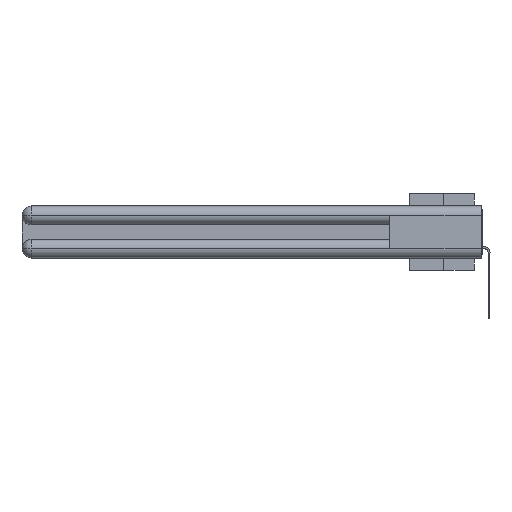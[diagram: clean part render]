
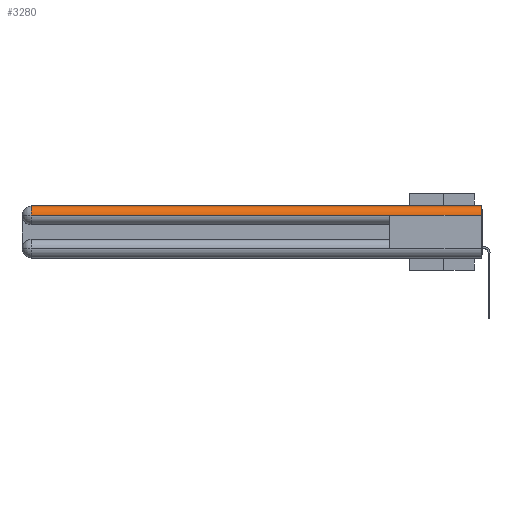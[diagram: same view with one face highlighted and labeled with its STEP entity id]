
A CAD part, left-side view. The second image highlights one B-rep face of the part: STEP entity #3280.
In plain terms, the highlighted cylindrical face has radius 1.562 mm (diameter 3.124 mm), a partial arc.
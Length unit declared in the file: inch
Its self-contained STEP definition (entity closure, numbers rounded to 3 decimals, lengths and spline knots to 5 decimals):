
#3280 = ADVANCED_FACE ( 'NONE', ( #16527 ), #18516, .T. ) ;
#3912 = ORIENTED_EDGE ( 'NONE', *, *, #4350, .F. ) ;
#4350 = EDGE_CURVE ( 'NONE', #36509, #22340, #38670, .T. ) ;
#5011 = DIRECTION ( 'NONE',  ( 0., -1., 0. ) ) ;
#5076 = VERTEX_POINT ( 'NONE', #14578 ) ;
#5189 = CARTESIAN_POINT ( 'NONE',  ( 0.0615, 2.94, 0. ) ) ;
#5241 = EDGE_CURVE ( 'NONE', #19698, #28461, #25313, .T. ) ;
#12131 = ORIENTED_EDGE ( 'NONE', *, *, #29637, .T. ) ;
#14134 = AXIS2_PLACEMENT_3D ( 'NONE', #31324, #15736, #18638 ) ;
#14578 = CARTESIAN_POINT ( 'NONE',  ( 0., 2.94, -0.0615 ) ) ;
#14628 = DIRECTION ( 'NONE',  ( 0., 1., 0. ) ) ;
#15383 = DIRECTION ( 'NONE',  ( 0., -1., 0. ) ) ;
#15409 = CIRCLE ( 'NONE', #25533, 0.0615 ) ;
#15736 = DIRECTION ( 'NONE',  ( 0., 1., 0. ) ) ;
#16182 = ORIENTED_EDGE ( 'NONE', *, *, #5241, .F. ) ;
#16527 = FACE_OUTER_BOUND ( 'NONE', #37663, .T. ) ;
#17567 = CARTESIAN_POINT ( 'NONE',  ( 0., 0.6, -0.0615 ) ) ;
#18488 = CARTESIAN_POINT ( 'NONE',  ( 0., 0., -0.0615 ) ) ;
#18516 = CYLINDRICAL_SURFACE ( 'NONE', #14134, 0.0615 ) ;
#18638 = DIRECTION ( 'NONE',  ( 0., 0., 1. ) ) ;
#18880 = VECTOR ( 'NONE', #15383, 39.37008 ) ;
#18882 = VECTOR ( 'NONE', #5011, 39.37008 ) ;
#19698 = VERTEX_POINT ( 'NONE', #5189 ) ;
#20420 = CARTESIAN_POINT ( 'NONE',  ( 0.0615, 0., 0. ) ) ;
#22340 = VERTEX_POINT ( 'NONE', #17567 ) ;
#22409 = EDGE_CURVE ( 'NONE', #28461, #36509, #15409, .T. ) ;
#22964 = CARTESIAN_POINT ( 'NONE',  ( 0.0615, 2.94, -0.0615 ) ) ;
#25313 = LINE ( 'NONE', #34278, #18880 ) ;
#25533 = AXIS2_PLACEMENT_3D ( 'NONE', #27645, #33833, #37296 ) ;
#26119 = CIRCLE ( 'NONE', #39252, 0.0615 ) ;
#26843 = CARTESIAN_POINT ( 'NONE',  ( 0., 3., -0.0615 ) ) ;
#27194 = CARTESIAN_POINT ( 'NONE',  ( 0., 3., -0.0615 ) ) ;
#27645 = CARTESIAN_POINT ( 'NONE',  ( 0.0615, 0., -0.0615 ) ) ;
#28461 = VERTEX_POINT ( 'NONE', #20420 ) ;
#29436 = DIRECTION ( 'NONE',  ( 0., -1., 0. ) ) ;
#29637 = EDGE_CURVE ( 'NONE', #5076, #22340, #38120, .T. ) ;
#30359 = ORIENTED_EDGE ( 'NONE', *, *, #22409, .F. ) ;
#31324 = CARTESIAN_POINT ( 'NONE',  ( 0.0615, 0., -0.0615 ) ) ;
#31497 = EDGE_CURVE ( 'NONE', #19698, #5076, #26119, .T. ) ;
#32466 = DIRECTION ( 'NONE',  ( 0., 0., 1. ) ) ;
#33833 = DIRECTION ( 'NONE',  ( 0., -1., 0. ) ) ;
#34278 = CARTESIAN_POINT ( 'NONE',  ( 0.0615, 0., 0. ) ) ;
#36509 = VERTEX_POINT ( 'NONE', #18488 ) ;
#36916 = ORIENTED_EDGE ( 'NONE', *, *, #31497, .T. ) ;
#37296 = DIRECTION ( 'NONE',  ( 1., 0., 0. ) ) ;
#37663 = EDGE_LOOP ( 'NONE', ( #16182, #36916, #12131, #3912, #30359 ) ) ;
#38120 = LINE ( 'NONE', #26843, #18882 ) ;
#38670 = LINE ( 'NONE', #27194, #40655 ) ;
#39252 = AXIS2_PLACEMENT_3D ( 'NONE', #22964, #29436, #32466 ) ;
#40655 = VECTOR ( 'NONE', #14628, 39.37008 ) ;
